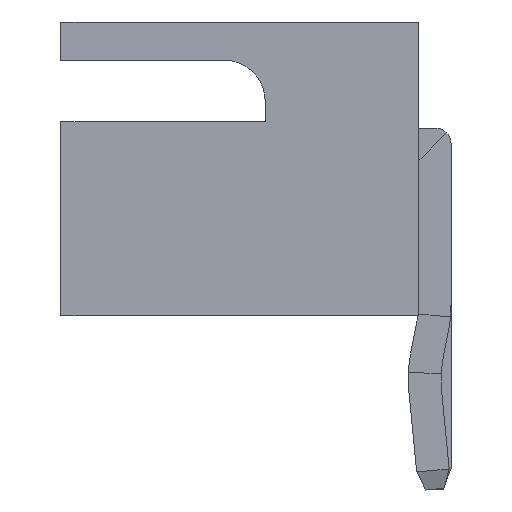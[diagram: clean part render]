
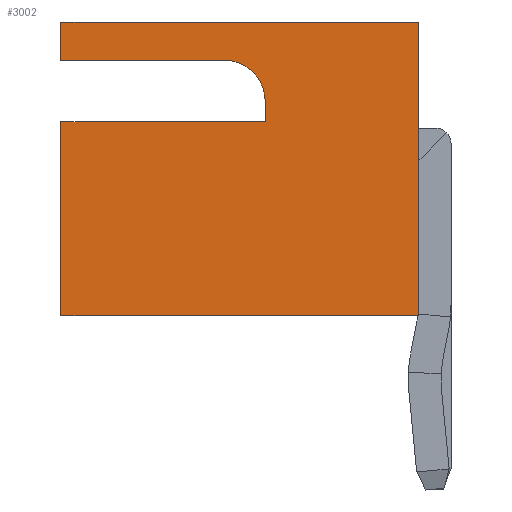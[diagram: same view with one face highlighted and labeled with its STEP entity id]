
A CAD part, left-side view. The second image highlights one B-rep face of the part: STEP entity #3002.
In plain terms, the highlighted planar face has unit normal (-1, 0, 0).
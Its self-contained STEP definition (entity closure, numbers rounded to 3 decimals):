
#2 = ORIENTED_EDGE ( 'NONE', *, *, #6290, .F. ) ;
#85 = VECTOR ( 'NONE', #6387, 1000. ) ;
#97 = AXIS2_PLACEMENT_3D ( 'NONE', #2075, #1264, #3405 ) ;
#244 = ORIENTED_EDGE ( 'NONE', *, *, #6890, .F. ) ;
#545 = VERTEX_POINT ( 'NONE', #1839 ) ;
#549 = EDGE_CURVE ( 'NONE', #8201, #3745, #1206, .T. ) ;
#707 = DIRECTION ( 'NONE',  ( 0., 0., 1. ) ) ;
#737 = VECTOR ( 'NONE', #6781, 1000. ) ;
#935 = EDGE_CURVE ( 'NONE', #545, #4208, #1275, .T. ) ;
#990 = CARTESIAN_POINT ( 'NONE',  ( -18.75, 7., -2.875 ) ) ;
#1010 = CARTESIAN_POINT ( 'NONE',  ( -18.75, 3.8, 2.125 ) ) ;
#1092 = VERTEX_POINT ( 'NONE', #4668 ) ;
#1144 = DIRECTION ( 'NONE',  ( 0., 0., -1. ) ) ;
#1206 = LINE ( 'NONE', #5788, #3494 ) ;
#1264 = DIRECTION ( 'NONE',  ( 1., 0., 0. ) ) ;
#1275 = LINE ( 'NONE', #5827, #85 ) ;
#1401 = FACE_OUTER_BOUND ( 'NONE', #8025, .T. ) ;
#1403 = ORIENTED_EDGE ( 'NONE', *, *, #5729, .T. ) ;
#1465 = LINE ( 'NONE', #990, #737 ) ;
#1499 = CARTESIAN_POINT ( 'NONE',  ( -18.75, 7., 0.925 ) ) ;
#1597 = ORIENTED_EDGE ( 'NONE', *, *, #5891, .T. ) ;
#1666 = VECTOR ( 'NONE', #6059, 1000. ) ;
#1700 = VECTOR ( 'NONE', #7027, 1000. ) ;
#1706 = ORIENTED_EDGE ( 'NONE', *, *, #7528, .F. ) ;
#1839 = CARTESIAN_POINT ( 'NONE',  ( -18.75, 7., 2.125 ) ) ;
#1877 = ORIENTED_EDGE ( 'NONE', *, *, #5742, .T. ) ;
#2075 = CARTESIAN_POINT ( 'NONE',  ( -18.75, 7., -2.875 ) ) ;
#2183 = LINE ( 'NONE', #2908, #1700 ) ;
#2546 = CARTESIAN_POINT ( 'NONE',  ( -18.75, 7., -2.875 ) ) ;
#2908 = CARTESIAN_POINT ( 'NONE',  ( -18.75, 7., 2.875 ) ) ;
#3002 = ADVANCED_FACE ( 'NONE', ( #1401 ), #7152, .F. ) ;
#3405 = DIRECTION ( 'NONE',  ( 0., 0., -1. ) ) ;
#3494 = VECTOR ( 'NONE', #8426, 1000. ) ;
#3582 = ORIENTED_EDGE ( 'NONE', *, *, #3635, .T. ) ;
#3620 = VECTOR ( 'NONE', #4616, 1000. ) ;
#3635 = EDGE_CURVE ( 'NONE', #1092, #6556, #6025, .T. ) ;
#3722 = CARTESIAN_POINT ( 'NONE',  ( -18.75, 3., 0.925 ) ) ;
#3745 = VERTEX_POINT ( 'NONE', #3722 ) ;
#4005 = LINE ( 'NONE', #5378, #6775 ) ;
#4118 = LINE ( 'NONE', #1499, #4708 ) ;
#4208 = VERTEX_POINT ( 'NONE', #1010 ) ;
#4447 = DIRECTION ( 'NONE',  ( 1., 0., 0. ) ) ;
#4616 = DIRECTION ( 'NONE',  ( 0., 0., 1. ) ) ;
#4668 = CARTESIAN_POINT ( 'NONE',  ( -18.75, 0., -2.875 ) ) ;
#4708 = VECTOR ( 'NONE', #4724, 1000. ) ;
#4724 = DIRECTION ( 'NONE',  ( 0., 1., 0. ) ) ;
#5253 = CARTESIAN_POINT ( 'NONE',  ( -18.75, 7., -2.875 ) ) ;
#5378 = CARTESIAN_POINT ( 'NONE',  ( -18.75, 7., -2.875 ) ) ;
#5532 = CARTESIAN_POINT ( 'NONE',  ( -18.75, 7., 2.875 ) ) ;
#5712 = CARTESIAN_POINT ( 'NONE',  ( -18.75, 0., 2.875 ) ) ;
#5729 = EDGE_CURVE ( 'NONE', #3745, #6039, #4118, .T. ) ;
#5742 = EDGE_CURVE ( 'NONE', #7515, #1092, #1465, .T. ) ;
#5788 = CARTESIAN_POINT ( 'NONE',  ( -18.75, 3., 1.325 ) ) ;
#5827 = CARTESIAN_POINT ( 'NONE',  ( -18.75, 7., 2.125 ) ) ;
#5891 = EDGE_CURVE ( 'NONE', #4208, #8201, #7037, .T. ) ;
#6025 = LINE ( 'NONE', #7403, #1666 ) ;
#6039 = VERTEX_POINT ( 'NONE', #7164 ) ;
#6059 = DIRECTION ( 'NONE',  ( 0., 0., 1. ) ) ;
#6290 = EDGE_CURVE ( 'NONE', #545, #6937, #4005, .T. ) ;
#6387 = DIRECTION ( 'NONE',  ( 0., -1., 0. ) ) ;
#6556 = VERTEX_POINT ( 'NONE', #5712 ) ;
#6775 = VECTOR ( 'NONE', #707, 1000. ) ;
#6781 = DIRECTION ( 'NONE',  ( 0., -1., 0. ) ) ;
#6789 = ORIENTED_EDGE ( 'NONE', *, *, #935, .T. ) ;
#6890 = EDGE_CURVE ( 'NONE', #6937, #6556, #2183, .T. ) ;
#6937 = VERTEX_POINT ( 'NONE', #5532 ) ;
#6960 = CARTESIAN_POINT ( 'NONE',  ( -18.75, 3.8, 1.325 ) ) ;
#7027 = DIRECTION ( 'NONE',  ( 0., -1., 0. ) ) ;
#7037 = CIRCLE ( 'NONE', #8146, 0.8 ) ;
#7152 = PLANE ( 'NONE',  #97 ) ;
#7164 = CARTESIAN_POINT ( 'NONE',  ( -18.75, 7., 0.925 ) ) ;
#7403 = CARTESIAN_POINT ( 'NONE',  ( -18.75, 0., -2.875 ) ) ;
#7515 = VERTEX_POINT ( 'NONE', #2546 ) ;
#7528 = EDGE_CURVE ( 'NONE', #7515, #6039, #8399, .T. ) ;
#8003 = CARTESIAN_POINT ( 'NONE',  ( -18.75, 3., 1.325 ) ) ;
#8025 = EDGE_LOOP ( 'NONE', ( #2, #6789, #1597, #8271, #1403, #1706, #1877, #3582, #244 ) ) ;
#8146 = AXIS2_PLACEMENT_3D ( 'NONE', #6960, #4447, #1144 ) ;
#8201 = VERTEX_POINT ( 'NONE', #8003 ) ;
#8271 = ORIENTED_EDGE ( 'NONE', *, *, #549, .T. ) ;
#8399 = LINE ( 'NONE', #5253, #3620 ) ;
#8426 = DIRECTION ( 'NONE',  ( 0., 0., -1. ) ) ;
